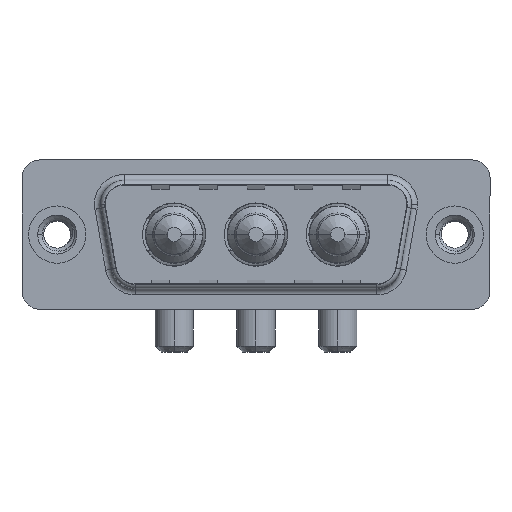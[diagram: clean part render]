
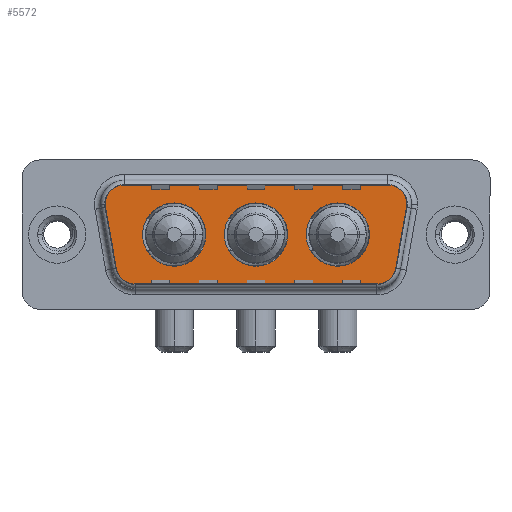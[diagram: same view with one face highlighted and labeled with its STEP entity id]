
A CAD part, top view. The second image highlights one B-rep face of the part: STEP entity #5572.
In plain terms, the highlighted planar face has unit normal (0, 0, 1).
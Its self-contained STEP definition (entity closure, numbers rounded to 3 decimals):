
#90 = VERTEX_POINT ( 'NONE', #8873 ) ;
#100 = DIRECTION ( 'NONE',  ( 0., 0., 1. ) ) ;
#148 = CIRCLE ( 'NONE', #3060, 2.65 ) ;
#198 = ORIENTED_EDGE ( 'NONE', *, *, #7640, .F. ) ;
#255 = AXIS2_PLACEMENT_3D ( 'NONE', #3282, #100, #12186 ) ;
#271 = CARTESIAN_POINT ( 'NONE',  ( 28.836, -3.247, 0. ) ) ;
#298 = ORIENTED_EDGE ( 'NONE', *, *, #11968, .T. ) ;
#300 = EDGE_CURVE ( 'NONE', #9814, #11183, #8193, .T. ) ;
#336 = CARTESIAN_POINT ( 'NONE',  ( 29.859, 2.553, 0. ) ) ;
#373 = DIRECTION ( 'NONE',  ( 1., 0., 0. ) ) ;
#497 = EDGE_CURVE ( 'NONE', #7592, #12592, #5146, .T. ) ;
#632 = VERTEX_POINT ( 'NONE', #1242 ) ;
#644 = CARTESIAN_POINT ( 'NONE',  ( 6.434, -4.9, 0. ) ) ;
#807 = EDGE_CURVE ( 'NONE', #11183, #5132, #7918, .T. ) ;
#825 = CARTESIAN_POINT ( 'NONE',  ( 26.866, -4.9, 0. ) ) ;
#829 = CIRCLE ( 'NONE', #8118, 2. ) ;
#868 = ORIENTED_EDGE ( 'NONE', *, *, #9899, .F. ) ;
#908 = CIRCLE ( 'NONE', #2570, 2.65 ) ;
#1026 = VECTOR ( 'NONE', #6072, 1000. ) ;
#1089 = CARTESIAN_POINT ( 'NONE',  ( 5.411, 4.9, 0. ) ) ;
#1166 = ORIENTED_EDGE ( 'NONE', *, *, #807, .T. ) ;
#1236 = DIRECTION ( 'NONE',  ( 1., 0., 0. ) ) ;
#1242 = CARTESIAN_POINT ( 'NONE',  ( 14., 0., 0. ) ) ;
#1246 = DIRECTION ( 'NONE',  ( 1., 0., 0. ) ) ;
#1352 = EDGE_LOOP ( 'NONE', ( #10258, #9915 ) ) ;
#1435 = ORIENTED_EDGE ( 'NONE', *, *, #4508, .T. ) ;
#1484 = EDGE_CURVE ( 'NONE', #3335, #632, #2500, .T. ) ;
#1608 = VERTEX_POINT ( 'NONE', #644 ) ;
#1768 = CIRCLE ( 'NONE', #9072, 2.65 ) ;
#1794 = ORIENTED_EDGE ( 'NONE', *, *, #12450, .F. ) ;
#1837 = EDGE_LOOP ( 'NONE', ( #198, #1794 ) ) ;
#1875 = AXIS2_PLACEMENT_3D ( 'NONE', #8479, #11294, #6312 ) ;
#2007 = DIRECTION ( 'NONE',  ( 1., 0., 0. ) ) ;
#2025 = CARTESIAN_POINT ( 'NONE',  ( 4.464, -3.247, 0. ) ) ;
#2497 = EDGE_CURVE ( 'NONE', #11612, #7592, #829, .T. ) ;
#2500 = CIRCLE ( 'NONE', #12526, 2.65 ) ;
#2570 = AXIS2_PLACEMENT_3D ( 'NONE', #11974, #5018, #9961 ) ;
#2725 = CARTESIAN_POINT ( 'NONE',  ( 3.441, 2.553, 0. ) ) ;
#2817 = CIRCLE ( 'NONE', #8502, 2.65 ) ;
#2830 = AXIS2_PLACEMENT_3D ( 'NONE', #11814, #4859, #8880 ) ;
#2837 = FACE_BOUND ( 'NONE', #1837, .T. ) ;
#3038 = CARTESIAN_POINT ( 'NONE',  ( 16.65, 0., 0. ) ) ;
#3060 = AXIS2_PLACEMENT_3D ( 'NONE', #8240, #4106, #1236 ) ;
#3180 = ORIENTED_EDGE ( 'NONE', *, *, #12156, .T. ) ;
#3208 = DIRECTION ( 'NONE',  ( 0., 0., 1. ) ) ;
#3282 = CARTESIAN_POINT ( 'NONE',  ( 27.889, 2.9, 0. ) ) ;
#3335 = VERTEX_POINT ( 'NONE', #11348 ) ;
#3415 = CARTESIAN_POINT ( 'NONE',  ( 7.15, 0., 0. ) ) ;
#3456 = EDGE_LOOP ( 'NONE', ( #5398, #4693, #298, #3180, #12608, #1166, #12328, #8912, #1435 ) ) ;
#3704 = DIRECTION ( 'NONE',  ( 0.174, -0.985, 0. ) ) ;
#3890 = PLANE ( 'NONE',  #5504 ) ;
#4074 = CIRCLE ( 'NONE', #2830, 2. ) ;
#4106 = DIRECTION ( 'NONE',  ( 0., 0., 1. ) ) ;
#4114 = CARTESIAN_POINT ( 'NONE',  ( 29.859, 2.553, 0. ) ) ;
#4346 = VERTEX_POINT ( 'NONE', #8062 ) ;
#4375 = DIRECTION ( 'NONE',  ( 1., 0., 0. ) ) ;
#4508 = EDGE_CURVE ( 'NONE', #1608, #11612, #4631, .T. ) ;
#4631 = LINE ( 'NONE', #5493, #5669 ) ;
#4693 = ORIENTED_EDGE ( 'NONE', *, *, #497, .T. ) ;
#4791 = DIRECTION ( 'NONE',  ( 0., 0., 1. ) ) ;
#4859 = DIRECTION ( 'NONE',  ( 0., 0., 1. ) ) ;
#5018 = DIRECTION ( 'NONE',  ( 0., 0., 1. ) ) ;
#5132 = VERTEX_POINT ( 'NONE', #12734 ) ;
#5146 = LINE ( 'NONE', #336, #1026 ) ;
#5159 = DIRECTION ( 'NONE',  ( 0., 0., 1. ) ) ;
#5398 = ORIENTED_EDGE ( 'NONE', *, *, #2497, .T. ) ;
#5493 = CARTESIAN_POINT ( 'NONE',  ( 6.434, -4.9, 0. ) ) ;
#5504 = AXIS2_PLACEMENT_3D ( 'NONE', #9667, #11864, #10902 ) ;
#5572 = ADVANCED_FACE ( 'NONE', ( #5843, #8876, #2837, #6831 ), #3890, .T. ) ;
#5606 = VECTOR ( 'NONE', #7205, 1000. ) ;
#5618 = VERTEX_POINT ( 'NONE', #12119 ) ;
#5653 = ORIENTED_EDGE ( 'NONE', *, *, #1484, .F. ) ;
#5669 = VECTOR ( 'NONE', #9634, 1000. ) ;
#5737 = CARTESIAN_POINT ( 'NONE',  ( 23.5, 0., 0. ) ) ;
#5843 = FACE_BOUND ( 'NONE', #9410, .T. ) ;
#5882 = CIRCLE ( 'NONE', #255, 2. ) ;
#5932 = VERTEX_POINT ( 'NONE', #3415 ) ;
#5979 = CARTESIAN_POINT ( 'NONE',  ( 27.889, 4.9, 0. ) ) ;
#6072 = DIRECTION ( 'NONE',  ( 0.174, 0.985, 0. ) ) ;
#6223 = CARTESIAN_POINT ( 'NONE',  ( 5.411, 4.9, 0. ) ) ;
#6312 = DIRECTION ( 'NONE',  ( 1., 0., 0. ) ) ;
#6524 = CIRCLE ( 'NONE', #9459, 2. ) ;
#6831 = FACE_OUTER_BOUND ( 'NONE', #3456, .T. ) ;
#6923 = EDGE_CURVE ( 'NONE', #9308, #1608, #4074, .T. ) ;
#7205 = DIRECTION ( 'NONE',  ( -1., 0., 0. ) ) ;
#7341 = DIRECTION ( 'NONE',  ( 0., 0., 1. ) ) ;
#7592 = VERTEX_POINT ( 'NONE', #271 ) ;
#7640 = EDGE_CURVE ( 'NONE', #7963, #5932, #148, .T. ) ;
#7918 = CIRCLE ( 'NONE', #1875, 2. ) ;
#7963 = VERTEX_POINT ( 'NONE', #8838 ) ;
#8062 = CARTESIAN_POINT ( 'NONE',  ( 20.85, 0., 0. ) ) ;
#8118 = AXIS2_PLACEMENT_3D ( 'NONE', #12172, #3208, #4375 ) ;
#8193 = LINE ( 'NONE', #6223, #5606 ) ;
#8240 = CARTESIAN_POINT ( 'NONE',  ( 9.8, 0., 0. ) ) ;
#8392 = DIRECTION ( 'NONE',  ( -1., 0., 0. ) ) ;
#8479 = CARTESIAN_POINT ( 'NONE',  ( 5.411, 2.9, 0. ) ) ;
#8502 = AXIS2_PLACEMENT_3D ( 'NONE', #3038, #10181, #373 ) ;
#8751 = EDGE_CURVE ( 'NONE', #90, #4346, #908, .T. ) ;
#8838 = CARTESIAN_POINT ( 'NONE',  ( 12.45, 0., 0. ) ) ;
#8873 = CARTESIAN_POINT ( 'NONE',  ( 26.15, 0., 0. ) ) ;
#8876 = FACE_BOUND ( 'NONE', #1352, .T. ) ;
#8880 = DIRECTION ( 'NONE',  ( -1., 0., 0. ) ) ;
#8881 = CARTESIAN_POINT ( 'NONE',  ( 16.65, 0., 0. ) ) ;
#8912 = ORIENTED_EDGE ( 'NONE', *, *, #6923, .T. ) ;
#9072 = AXIS2_PLACEMENT_3D ( 'NONE', #5737, #11820, #2007 ) ;
#9308 = VERTEX_POINT ( 'NONE', #2025 ) ;
#9410 = EDGE_LOOP ( 'NONE', ( #5653, #868 ) ) ;
#9459 = AXIS2_PLACEMENT_3D ( 'NONE', #9649, #7341, #8392 ) ;
#9634 = DIRECTION ( 'NONE',  ( 1., 0., 0. ) ) ;
#9649 = CARTESIAN_POINT ( 'NONE',  ( 27.889, 2.9, 0. ) ) ;
#9652 = EDGE_CURVE ( 'NONE', #5132, #9308, #10532, .T. ) ;
#9667 = CARTESIAN_POINT ( 'NONE',  ( 26.866, -2.9, 0. ) ) ;
#9758 = EDGE_CURVE ( 'NONE', #4346, #90, #1768, .T. ) ;
#9814 = VERTEX_POINT ( 'NONE', #5979 ) ;
#9899 = EDGE_CURVE ( 'NONE', #632, #3335, #2817, .T. ) ;
#9915 = ORIENTED_EDGE ( 'NONE', *, *, #9758, .F. ) ;
#9961 = DIRECTION ( 'NONE',  ( 1., 0., 0. ) ) ;
#10026 = CARTESIAN_POINT ( 'NONE',  ( 9.8, 0., 0. ) ) ;
#10181 = DIRECTION ( 'NONE',  ( 0., 0., 1. ) ) ;
#10258 = ORIENTED_EDGE ( 'NONE', *, *, #8751, .F. ) ;
#10532 = LINE ( 'NONE', #2725, #11030 ) ;
#10902 = DIRECTION ( 'NONE',  ( 1., 0., 0. ) ) ;
#11030 = VECTOR ( 'NONE', #3704, 1000. ) ;
#11121 = CIRCLE ( 'NONE', #12157, 2.65 ) ;
#11183 = VERTEX_POINT ( 'NONE', #1089 ) ;
#11294 = DIRECTION ( 'NONE',  ( 0., 0., 1. ) ) ;
#11348 = CARTESIAN_POINT ( 'NONE',  ( 19.3, 0., 0. ) ) ;
#11612 = VERTEX_POINT ( 'NONE', #825 ) ;
#11814 = CARTESIAN_POINT ( 'NONE',  ( 6.434, -2.9, 0. ) ) ;
#11820 = DIRECTION ( 'NONE',  ( 0., 0., 1. ) ) ;
#11864 = DIRECTION ( 'NONE',  ( 0., 0., 1. ) ) ;
#11968 = EDGE_CURVE ( 'NONE', #12592, #5618, #5882, .T. ) ;
#11974 = CARTESIAN_POINT ( 'NONE',  ( 23.5, 0., 0. ) ) ;
#12119 = CARTESIAN_POINT ( 'NONE',  ( 29.889, 2.9, 0. ) ) ;
#12156 = EDGE_CURVE ( 'NONE', #5618, #9814, #6524, .T. ) ;
#12157 = AXIS2_PLACEMENT_3D ( 'NONE', #10026, #5159, #1246 ) ;
#12172 = CARTESIAN_POINT ( 'NONE',  ( 26.866, -2.9, 0. ) ) ;
#12186 = DIRECTION ( 'NONE',  ( -1., 0., 0. ) ) ;
#12328 = ORIENTED_EDGE ( 'NONE', *, *, #9652, .T. ) ;
#12450 = EDGE_CURVE ( 'NONE', #5932, #7963, #11121, .T. ) ;
#12526 = AXIS2_PLACEMENT_3D ( 'NONE', #8881, #4791, #12858 ) ;
#12592 = VERTEX_POINT ( 'NONE', #4114 ) ;
#12608 = ORIENTED_EDGE ( 'NONE', *, *, #300, .T. ) ;
#12734 = CARTESIAN_POINT ( 'NONE',  ( 3.441, 2.553, 0. ) ) ;
#12858 = DIRECTION ( 'NONE',  ( 1., 0., 0. ) ) ;
